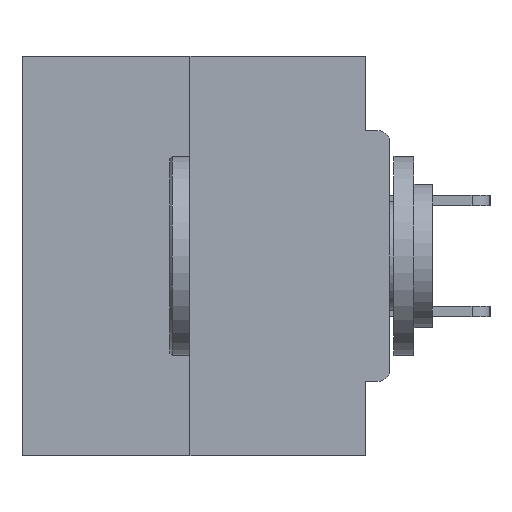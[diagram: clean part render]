
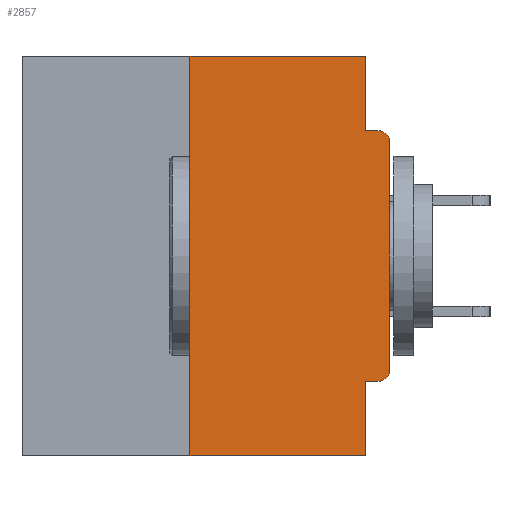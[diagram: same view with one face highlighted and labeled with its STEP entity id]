
A CAD part, left-side view. The second image highlights one B-rep face of the part: STEP entity #2857.
In plain terms, the highlighted planar face has unit normal (-1, 0, 0).
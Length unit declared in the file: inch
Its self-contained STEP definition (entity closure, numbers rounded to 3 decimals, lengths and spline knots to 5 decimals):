
#529 = DIRECTION ( 'NONE',  ( 0., -1., 0. ) ) ;
#613 = VERTEX_POINT ( 'NONE', #17692 ) ;
#1244 = CARTESIAN_POINT ( 'NONE',  ( 0., 0.031, -0.5 ) ) ;
#1551 = VERTEX_POINT ( 'NONE', #17254 ) ;
#1879 = CARTESIAN_POINT ( 'NONE',  ( 0., 0.031, -0.4065 ) ) ;
#2060 = ORIENTED_EDGE ( 'NONE', *, *, #12214, .F. ) ;
#2380 = VERTEX_POINT ( 'NONE', #1879 ) ;
#2746 = VERTEX_POINT ( 'NONE', #1244 ) ;
#2754 = CARTESIAN_POINT ( 'NONE',  ( 0., 0.46, 0. ) ) ;
#2857 = ADVANCED_FACE ( 'NONE', ( #8030 ), #11369, .F. ) ;
#3209 = DIRECTION ( 'NONE',  ( 0., 0., -1. ) ) ;
#4250 = AXIS2_PLACEMENT_3D ( 'NONE', #16355, #21769, #18921 ) ;
#4566 = VERTEX_POINT ( 'NONE', #5871 ) ;
#4585 = CARTESIAN_POINT ( 'NONE',  ( 0., 0.031, -0.5 ) ) ;
#5358 = CARTESIAN_POINT ( 'NONE',  ( 0., 0., 0. ) ) ;
#5515 = VECTOR ( 'NONE', #529, 39.37008 ) ;
#5674 = VERTEX_POINT ( 'NONE', #24946 ) ;
#5864 = CARTESIAN_POINT ( 'NONE',  ( 0., 0., -0.0935 ) ) ;
#5871 = CARTESIAN_POINT ( 'NONE',  ( 0., 0.031, -0.0935 ) ) ;
#6549 = VECTOR ( 'NONE', #13118, 39.37008 ) ;
#7657 = CIRCLE ( 'NONE', #4250, 0.015 ) ;
#8030 = FACE_OUTER_BOUND ( 'NONE', #19771, .T. ) ;
#8194 = LINE ( 'NONE', #5358, #6549 ) ;
#8350 = DIRECTION ( 'NONE',  ( -1., 0., 0. ) ) ;
#10806 = EDGE_CURVE ( 'NONE', #5674, #4566, #28254, .T. ) ;
#11369 = PLANE ( 'NONE',  #27108 ) ;
#11454 = ORIENTED_EDGE ( 'NONE', *, *, #18974, .T. ) ;
#11753 = VECTOR ( 'NONE', #28488, 39.37008 ) ;
#12214 = EDGE_CURVE ( 'NONE', #4566, #1551, #21392, .T. ) ;
#12661 = DIRECTION ( 'NONE',  ( 0., 0., 1. ) ) ;
#12706 = CARTESIAN_POINT ( 'NONE',  ( 0., 0.031, 0. ) ) ;
#12743 = VECTOR ( 'NONE', #19349, 39.37008 ) ;
#12836 = LINE ( 'NONE', #2754, #23148 ) ;
#13118 = DIRECTION ( 'NONE',  ( 0., 0., 1. ) ) ;
#13406 = CARTESIAN_POINT ( 'NONE',  ( 0., 0., -0.1085 ) ) ;
#13416 = CARTESIAN_POINT ( 'NONE',  ( 0., 0.015, -0.1085 ) ) ;
#13884 = VECTOR ( 'NONE', #14913, 39.37008 ) ;
#13907 = CARTESIAN_POINT ( 'NONE',  ( 0., 0.46, 0. ) ) ;
#14074 = EDGE_CURVE ( 'NONE', #613, #2746, #18515, .T. ) ;
#14716 = DIRECTION ( 'NONE',  ( 0., 0., -1. ) ) ;
#14757 = VECTOR ( 'NONE', #12661, 39.37008 ) ;
#14913 = DIRECTION ( 'NONE',  ( 0., 0., -1. ) ) ;
#15168 = ORIENTED_EDGE ( 'NONE', *, *, #29747, .T. ) ;
#15670 = ORIENTED_EDGE ( 'NONE', *, *, #31300, .F. ) ;
#15879 = AXIS2_PLACEMENT_3D ( 'NONE', #13416, #8350, #3209 ) ;
#16032 = EDGE_CURVE ( 'NONE', #21884, #1551, #21918, .T. ) ;
#16355 = CARTESIAN_POINT ( 'NONE',  ( 0., 0.015, -0.3915 ) ) ;
#16570 = DIRECTION ( 'NONE',  ( 0., 0., -1. ) ) ;
#16798 = CARTESIAN_POINT ( 'NONE',  ( 0., 0., -0.4065 ) ) ;
#16804 = ORIENTED_EDGE ( 'NONE', *, *, #16032, .T. ) ;
#17254 = CARTESIAN_POINT ( 'NONE',  ( 0., 0.015, -0.0935 ) ) ;
#17507 = VERTEX_POINT ( 'NONE', #23715 ) ;
#17692 = CARTESIAN_POINT ( 'NONE',  ( 0., 0.25, -0.5 ) ) ;
#17822 = CARTESIAN_POINT ( 'NONE',  ( 0., 0.46, -0.5 ) ) ;
#17916 = LINE ( 'NONE', #16798, #12743 ) ;
#18515 = LINE ( 'NONE', #17822, #11753 ) ;
#18579 = ORIENTED_EDGE ( 'NONE', *, *, #14074, .T. ) ;
#18921 = DIRECTION ( 'NONE',  ( 0., 0., -1. ) ) ;
#18974 = EDGE_CURVE ( 'NONE', #27763, #28109, #7657, .T. ) ;
#19349 = DIRECTION ( 'NONE',  ( 0., 1., 0. ) ) ;
#19771 = EDGE_LOOP ( 'NONE', ( #15670, #26765, #18579, #25631, #30724, #11454, #15168, #16804, #2060, #23883 ) ) ;
#21392 = LINE ( 'NONE', #5864, #5515 ) ;
#21769 = DIRECTION ( 'NONE',  ( -1., 0., 0. ) ) ;
#21884 = VERTEX_POINT ( 'NONE', #13406 ) ;
#21918 = CIRCLE ( 'NONE', #15879, 0.015 ) ;
#22535 = CARTESIAN_POINT ( 'NONE',  ( 0., 0.015, -0.4065 ) ) ;
#23148 = VECTOR ( 'NONE', #28327, 39.37008 ) ;
#23715 = CARTESIAN_POINT ( 'NONE',  ( 0., 0.25, 0. ) ) ;
#23883 = ORIENTED_EDGE ( 'NONE', *, *, #10806, .F. ) ;
#24946 = CARTESIAN_POINT ( 'NONE',  ( 0., 0.031, 0. ) ) ;
#25631 = ORIENTED_EDGE ( 'NONE', *, *, #32878, .F. ) ;
#26765 = ORIENTED_EDGE ( 'NONE', *, *, #32426, .F. ) ;
#27108 = AXIS2_PLACEMENT_3D ( 'NONE', #13907, #31701, #16570 ) ;
#27445 = LINE ( 'NONE', #4585, #13884 ) ;
#27763 = VERTEX_POINT ( 'NONE', #22535 ) ;
#28109 = VERTEX_POINT ( 'NONE', #31421 ) ;
#28216 = CARTESIAN_POINT ( 'NONE',  ( 0., 0.25, 0. ) ) ;
#28254 = LINE ( 'NONE', #12706, #29458 ) ;
#28327 = DIRECTION ( 'NONE',  ( 0., -1., 0. ) ) ;
#28488 = DIRECTION ( 'NONE',  ( 0., -1., 0. ) ) ;
#29068 = LINE ( 'NONE', #28216, #14757 ) ;
#29458 = VECTOR ( 'NONE', #14716, 39.37008 ) ;
#29747 = EDGE_CURVE ( 'NONE', #28109, #21884, #8194, .T. ) ;
#30724 = ORIENTED_EDGE ( 'NONE', *, *, #32835, .F. ) ;
#31300 = EDGE_CURVE ( 'NONE', #17507, #5674, #12836, .T. ) ;
#31421 = CARTESIAN_POINT ( 'NONE',  ( 0., 0., -0.3915 ) ) ;
#31701 = DIRECTION ( 'NONE',  ( 1., 0., 0. ) ) ;
#32426 = EDGE_CURVE ( 'NONE', #613, #17507, #29068, .T. ) ;
#32835 = EDGE_CURVE ( 'NONE', #27763, #2380, #17916, .T. ) ;
#32878 = EDGE_CURVE ( 'NONE', #2380, #2746, #27445, .T. ) ;
